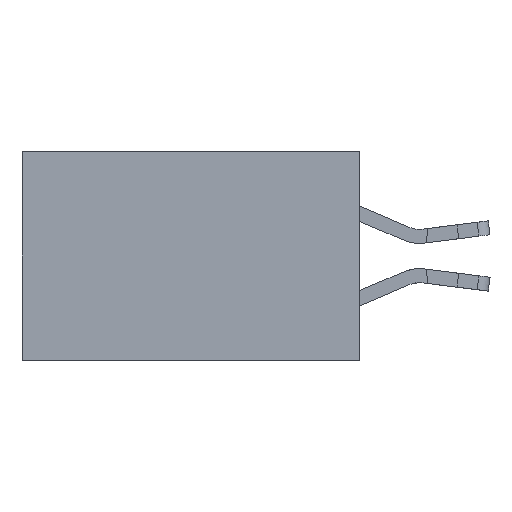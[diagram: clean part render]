
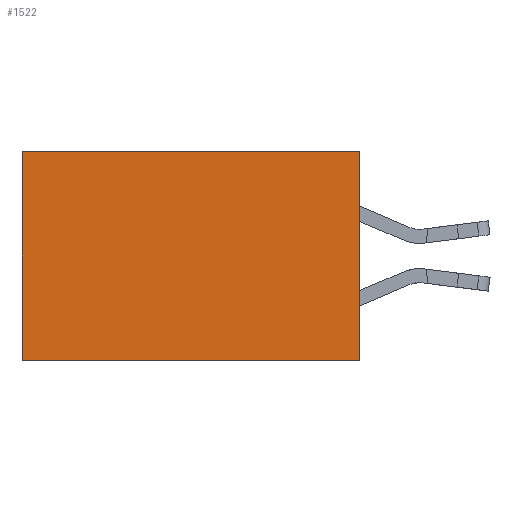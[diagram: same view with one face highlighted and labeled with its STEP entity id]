
A CAD part, left-side view. The second image highlights one B-rep face of the part: STEP entity #1522.
In plain terms, the highlighted planar face has unit normal (-1, 0, 0).
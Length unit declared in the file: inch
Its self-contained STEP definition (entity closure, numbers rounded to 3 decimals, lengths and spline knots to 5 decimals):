
#154 = EDGE_CURVE ( 'NONE', #17513, #17129, #6053, .T. ) ;
#295 = CARTESIAN_POINT ( 'NONE',  ( 0.2875, 0.6, -0.37 ) ) ;
#352 = LINE ( 'NONE', #10779, #9606 ) ;
#877 = ORIENTED_EDGE ( 'NONE', *, *, #3397, .T. ) ;
#1168 = DIRECTION ( 'NONE',  ( 1., 0., 0. ) ) ;
#1522 = ADVANCED_FACE ( 'NONE', ( #4347 ), #11605, .F. ) ;
#1787 = CARTESIAN_POINT ( 'NONE',  ( 0.2875, 0.6, 0. ) ) ;
#3397 = EDGE_CURVE ( 'NONE', #17129, #6075, #352, .T. ) ;
#4347 = FACE_OUTER_BOUND ( 'NONE', #8895, .T. ) ;
#4982 = DIRECTION ( 'NONE',  ( 0., 1., 0. ) ) ;
#6053 = LINE ( 'NONE', #18069, #18748 ) ;
#6075 = VERTEX_POINT ( 'NONE', #295 ) ;
#6878 = EDGE_CURVE ( 'NONE', #17351, #6075, #20870, .T. ) ;
#8298 = CARTESIAN_POINT ( 'NONE',  ( 0.2875, 0., -0.37 ) ) ;
#8895 = EDGE_LOOP ( 'NONE', ( #877, #19720, #11606, #10439 ) ) ;
#9606 = VECTOR ( 'NONE', #14299, 39.37008 ) ;
#10439 = ORIENTED_EDGE ( 'NONE', *, *, #154, .T. ) ;
#10663 = CARTESIAN_POINT ( 'NONE',  ( 0.2875, 0., 0. ) ) ;
#10779 = CARTESIAN_POINT ( 'NONE',  ( 0.2875, 0.6, 0. ) ) ;
#11605 = PLANE ( 'NONE',  #18206 ) ;
#11606 = ORIENTED_EDGE ( 'NONE', *, *, #16614, .F. ) ;
#11822 = LINE ( 'NONE', #15582, #15611 ) ;
#14163 = DIRECTION ( 'NONE',  ( 0., 0., -1. ) ) ;
#14299 = DIRECTION ( 'NONE',  ( 0., 0., -1. ) ) ;
#14626 = CARTESIAN_POINT ( 'NONE',  ( 0.2875, 0., 0. ) ) ;
#15582 = CARTESIAN_POINT ( 'NONE',  ( 0.2875, 0., 0. ) ) ;
#15611 = VECTOR ( 'NONE', #17233, 39.37008 ) ;
#16444 = VECTOR ( 'NONE', #4982, 39.37008 ) ;
#16614 = EDGE_CURVE ( 'NONE', #17513, #17351, #11822, .T. ) ;
#17129 = VERTEX_POINT ( 'NONE', #1787 ) ;
#17233 = DIRECTION ( 'NONE',  ( 0., 0., -1. ) ) ;
#17351 = VERTEX_POINT ( 'NONE', #20848 ) ;
#17513 = VERTEX_POINT ( 'NONE', #14626 ) ;
#18069 = CARTESIAN_POINT ( 'NONE',  ( 0.2875, 0., 0. ) ) ;
#18206 = AXIS2_PLACEMENT_3D ( 'NONE', #10663, #1168, #14163 ) ;
#18748 = VECTOR ( 'NONE', #19245, 39.37008 ) ;
#19245 = DIRECTION ( 'NONE',  ( 0., 1., 0. ) ) ;
#19720 = ORIENTED_EDGE ( 'NONE', *, *, #6878, .F. ) ;
#20848 = CARTESIAN_POINT ( 'NONE',  ( 0.2875, 0., -0.37 ) ) ;
#20870 = LINE ( 'NONE', #8298, #16444 ) ;
